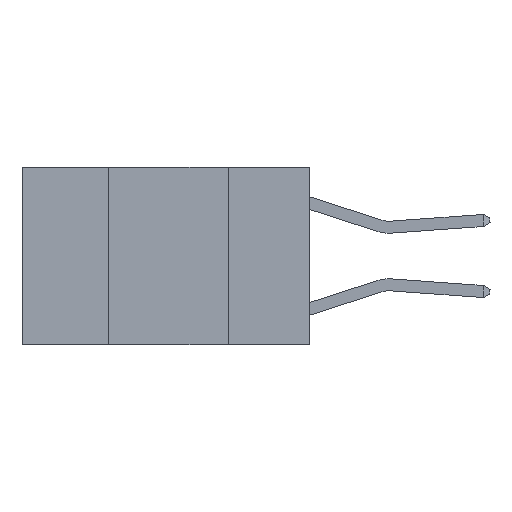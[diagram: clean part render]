
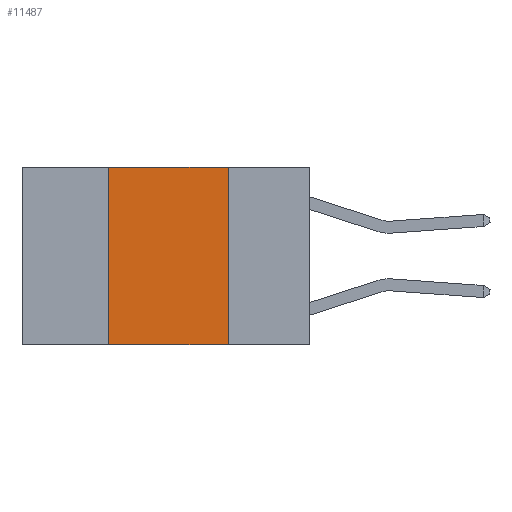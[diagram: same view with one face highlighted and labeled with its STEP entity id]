
A CAD part, left-side view. The second image highlights one B-rep face of the part: STEP entity #11487.
In plain terms, the highlighted planar face has unit normal (-1, 0, 0).
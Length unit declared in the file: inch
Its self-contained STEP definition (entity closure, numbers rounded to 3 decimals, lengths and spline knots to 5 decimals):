
#217 = CARTESIAN_POINT ( 'NONE',  ( 0., 0.6, -0.37 ) ) ;
#1322 = ORIENTED_EDGE ( 'NONE', *, *, #15487, .F. ) ;
#1840 = DIRECTION ( 'NONE',  ( 0., -1., 0. ) ) ;
#2106 = CARTESIAN_POINT ( 'NONE',  ( 0., 0.42, 0. ) ) ;
#2392 = ORIENTED_EDGE ( 'NONE', *, *, #8150, .T. ) ;
#2580 = DIRECTION ( 'NONE',  ( 0., 0., 1. ) ) ;
#3254 = VECTOR ( 'NONE', #1840, 39.37008 ) ;
#4397 = PLANE ( 'NONE',  #4541 ) ;
#4515 = ORIENTED_EDGE ( 'NONE', *, *, #13074, .F. ) ;
#4541 = AXIS2_PLACEMENT_3D ( 'NONE', #10766, #12102, #6609 ) ;
#4673 = CARTESIAN_POINT ( 'NONE',  ( 0., 0.42, -0.37 ) ) ;
#5088 = VERTEX_POINT ( 'NONE', #11761 ) ;
#5997 = VECTOR ( 'NONE', #7510, 39.37008 ) ;
#6609 = DIRECTION ( 'NONE',  ( 0., 0., -1. ) ) ;
#6896 = LINE ( 'NONE', #12659, #12298 ) ;
#7385 = VERTEX_POINT ( 'NONE', #2106 ) ;
#7510 = DIRECTION ( 'NONE',  ( 0., -1., 0. ) ) ;
#8150 = EDGE_CURVE ( 'NONE', #14548, #16200, #12883, .T. ) ;
#8212 = DIRECTION ( 'NONE',  ( 0., 0., -1. ) ) ;
#8500 = CARTESIAN_POINT ( 'NONE',  ( 0., 0.17, -0.37 ) ) ;
#10259 = CARTESIAN_POINT ( 'NONE',  ( 0., 0.6, 0. ) ) ;
#10766 = CARTESIAN_POINT ( 'NONE',  ( 0., 0.6, 0. ) ) ;
#11310 = LINE ( 'NONE', #12636, #15021 ) ;
#11487 = ADVANCED_FACE ( 'NONE', ( #17385 ), #4397, .F. ) ;
#11761 = CARTESIAN_POINT ( 'NONE',  ( 0., 0.17, 0. ) ) ;
#12102 = DIRECTION ( 'NONE',  ( 1., 0., 0. ) ) ;
#12298 = VECTOR ( 'NONE', #2580, 39.37008 ) ;
#12636 = CARTESIAN_POINT ( 'NONE',  ( 0., 0.17, 0. ) ) ;
#12659 = CARTESIAN_POINT ( 'NONE',  ( 0., 0.42, 0. ) ) ;
#12883 = LINE ( 'NONE', #217, #3254 ) ;
#13074 = EDGE_CURVE ( 'NONE', #14548, #7385, #6896, .T. ) ;
#13183 = LINE ( 'NONE', #10259, #5997 ) ;
#13465 = EDGE_CURVE ( 'NONE', #5088, #16200, #11310, .T. ) ;
#13978 = ORIENTED_EDGE ( 'NONE', *, *, #13465, .F. ) ;
#14548 = VERTEX_POINT ( 'NONE', #4673 ) ;
#15021 = VECTOR ( 'NONE', #8212, 39.37008 ) ;
#15487 = EDGE_CURVE ( 'NONE', #7385, #5088, #13183, .T. ) ;
#16014 = EDGE_LOOP ( 'NONE', ( #13978, #1322, #4515, #2392 ) ) ;
#16200 = VERTEX_POINT ( 'NONE', #8500 ) ;
#17385 = FACE_OUTER_BOUND ( 'NONE', #16014, .T. ) ;
